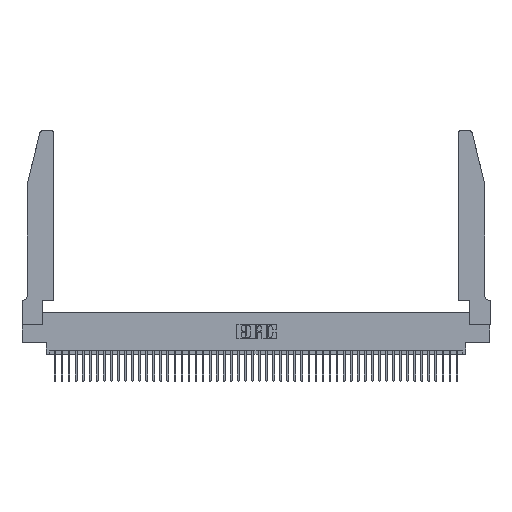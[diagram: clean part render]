
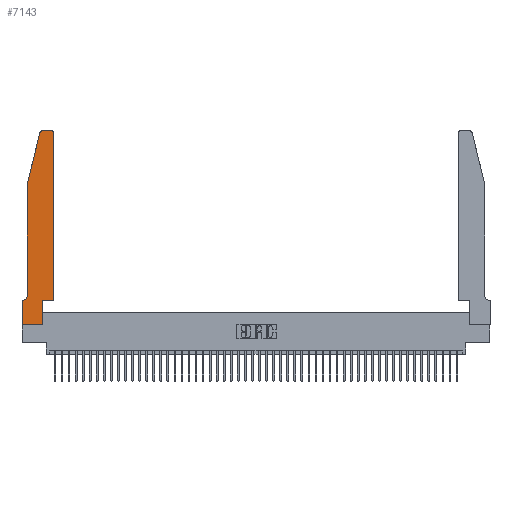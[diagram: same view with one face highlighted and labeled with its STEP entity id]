
A CAD part, top view. The second image highlights one B-rep face of the part: STEP entity #7143.
In plain terms, the highlighted planar face has unit normal (0, 0, 1).
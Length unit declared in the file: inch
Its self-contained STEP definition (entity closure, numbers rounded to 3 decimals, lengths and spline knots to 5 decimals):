
#429 = CARTESIAN_POINT ( 'NONE',  ( 0.4205, 2.75, 0.37 ) ) ;
#1253 = VERTEX_POINT ( 'NONE', #30717 ) ;
#1273 = CIRCLE ( 'NONE', #12332, 0.07 ) ;
#1673 = CARTESIAN_POINT ( 'NONE',  ( 0.0055, 0.42, 0.37 ) ) ;
#1912 = EDGE_CURVE ( 'NONE', #16612, #46207, #1273, .T. ) ;
#2440 = VECTOR ( 'NONE', #19115, 39.37008 ) ;
#2939 = DIRECTION ( 'NONE',  ( 0., -1., 0. ) ) ;
#3280 = CARTESIAN_POINT ( 'NONE',  ( 0.284, 2.75, 0.37 ) ) ;
#4116 = CARTESIAN_POINT ( 'NONE',  ( 0.4505, 0.35, 0.37 ) ) ;
#4199 = CARTESIAN_POINT ( 'NONE',  ( 0.25487, 2.72718, 0.37 ) ) ;
#4573 = EDGE_CURVE ( 'NONE', #17643, #6663, #27404, .T. ) ;
#4672 = EDGE_LOOP ( 'NONE', ( #35767, #28566, #30583, #44725, #23647, #26011, #35428, #19925, #42853, #39651, #7156, #32594 ) ) ;
#5201 = AXIS2_PLACEMENT_3D ( 'NONE', #37118, #32874, #29621 ) ;
#5440 = DIRECTION ( 'NONE',  ( 0., 0., -1. ) ) ;
#6197 = AXIS2_PLACEMENT_3D ( 'NONE', #39773, #47233, #17585 ) ;
#6663 = VERTEX_POINT ( 'NONE', #429 ) ;
#6762 = CARTESIAN_POINT ( 'NONE',  ( 0.2865, 0.35, 0.37 ) ) ;
#7143 = ADVANCED_FACE ( 'NONE', ( #12188 ), #13525, .T. ) ;
#7156 = ORIENTED_EDGE ( 'NONE', *, *, #31594, .T. ) ;
#7603 = DIRECTION ( 'NONE',  ( 1., 0., 0. ) ) ;
#8366 = VECTOR ( 'NONE', #16433, 39.37008 ) ;
#9317 = VECTOR ( 'NONE', #34750, 39.37008 ) ;
#11186 = EDGE_CURVE ( 'NONE', #46207, #47413, #20607, .T. ) ;
#12188 = FACE_OUTER_BOUND ( 'NONE', #4672, .T. ) ;
#12332 = AXIS2_PLACEMENT_3D ( 'NONE', #1673, #5440, #38867 ) ;
#12929 = LINE ( 'NONE', #4116, #2440 ) ;
#13467 = VECTOR ( 'NONE', #36139, 39.37008 ) ;
#13525 = PLANE ( 'NONE',  #6197 ) ;
#13780 = CARTESIAN_POINT ( 'NONE',  ( 0.0055, 0.35, 0.37 ) ) ;
#14168 = VECTOR ( 'NONE', #18924, 39.37008 ) ;
#14359 = CARTESIAN_POINT ( 'NONE',  ( 0., 0., 0.37 ) ) ;
#14623 = DIRECTION ( 'NONE',  ( -1., 0., 0. ) ) ;
#14666 = VERTEX_POINT ( 'NONE', #30146 ) ;
#14786 = CARTESIAN_POINT ( 'NONE',  ( 0.0755, 0.35, 0.37 ) ) ;
#14976 = LINE ( 'NONE', #14359, #25525 ) ;
#15584 = CARTESIAN_POINT ( 'NONE',  ( 0.4505, 2.72, 0.37 ) ) ;
#15757 = EDGE_CURVE ( 'NONE', #42245, #24651, #16914, .T. ) ;
#16433 = DIRECTION ( 'NONE',  ( 1., 0., 0. ) ) ;
#16612 = VERTEX_POINT ( 'NONE', #36038 ) ;
#16914 = LINE ( 'NONE', #26318, #9317 ) ;
#17342 = CARTESIAN_POINT ( 'NONE',  ( 0.0755, 2., 0.37 ) ) ;
#17585 = DIRECTION ( 'NONE',  ( 1., 0., 0. ) ) ;
#17643 = VERTEX_POINT ( 'NONE', #15584 ) ;
#17665 = VECTOR ( 'NONE', #14623, 39.37008 ) ;
#17861 = VECTOR ( 'NONE', #31596, 39.37008 ) ;
#18639 = VECTOR ( 'NONE', #28764, 39.37008 ) ;
#18731 = VERTEX_POINT ( 'NONE', #3280 ) ;
#18924 = DIRECTION ( 'NONE',  ( 0., -1., 0. ) ) ;
#19073 = EDGE_CURVE ( 'NONE', #14666, #42245, #43938, .T. ) ;
#19115 = DIRECTION ( 'NONE',  ( 1., 0., 0. ) ) ;
#19174 = LINE ( 'NONE', #35000, #17861 ) ;
#19593 = EDGE_CURVE ( 'NONE', #6663, #18731, #19174, .T. ) ;
#19721 = CARTESIAN_POINT ( 'NONE',  ( 0., 0., 0.37 ) ) ;
#19925 = ORIENTED_EDGE ( 'NONE', *, *, #19073, .T. ) ;
#20607 = LINE ( 'NONE', #14786, #17665 ) ;
#23597 = EDGE_CURVE ( 'NONE', #36610, #16612, #38091, .T. ) ;
#23647 = ORIENTED_EDGE ( 'NONE', *, *, #1912, .T. ) ;
#24651 = VERTEX_POINT ( 'NONE', #6762 ) ;
#25525 = VECTOR ( 'NONE', #2939, 39.37008 ) ;
#26011 = ORIENTED_EDGE ( 'NONE', *, *, #11186, .T. ) ;
#26318 = CARTESIAN_POINT ( 'NONE',  ( 0.2865, 0.35, 0.37 ) ) ;
#27404 = CIRCLE ( 'NONE', #38605, 0.03 ) ;
#28566 = ORIENTED_EDGE ( 'NONE', *, *, #35561, .T. ) ;
#28571 = LINE ( 'NONE', #17342, #18639 ) ;
#28764 = DIRECTION ( 'NONE',  ( -0.239, -0.971, 0. ) ) ;
#29621 = DIRECTION ( 'NONE',  ( 1., 0., 0. ) ) ;
#29978 = CARTESIAN_POINT ( 'NONE',  ( 0.4205, 2.72, 0.37 ) ) ;
#30146 = CARTESIAN_POINT ( 'NONE',  ( 0., 0., 0.37 ) ) ;
#30583 = ORIENTED_EDGE ( 'NONE', *, *, #41108, .T. ) ;
#30687 = CARTESIAN_POINT ( 'NONE',  ( 0.0755, 2., 0.37 ) ) ;
#30717 = CARTESIAN_POINT ( 'NONE',  ( 0.4505, 0.35, 0.37 ) ) ;
#31594 = EDGE_CURVE ( 'NONE', #1253, #17643, #40272, .T. ) ;
#31596 = DIRECTION ( 'NONE',  ( -1., 0., 0. ) ) ;
#32393 = CARTESIAN_POINT ( 'NONE',  ( 0.4505, 0.35, 0.37 ) ) ;
#32594 = ORIENTED_EDGE ( 'NONE', *, *, #4573, .T. ) ;
#32874 = DIRECTION ( 'NONE',  ( 0., 0., 1. ) ) ;
#34750 = DIRECTION ( 'NONE',  ( 0., 1., 0. ) ) ;
#34786 = CIRCLE ( 'NONE', #5201, 0.03 ) ;
#35000 = CARTESIAN_POINT ( 'NONE',  ( 0.2605, 2.75, 0.37 ) ) ;
#35352 = CARTESIAN_POINT ( 'NONE',  ( 0.2865, 0., 0.37 ) ) ;
#35428 = ORIENTED_EDGE ( 'NONE', *, *, #43652, .T. ) ;
#35561 = EDGE_CURVE ( 'NONE', #18731, #37104, #34786, .T. ) ;
#35767 = ORIENTED_EDGE ( 'NONE', *, *, #19593, .T. ) ;
#36038 = CARTESIAN_POINT ( 'NONE',  ( 0.0755, 0.42, 0.37 ) ) ;
#36139 = DIRECTION ( 'NONE',  ( 0., 1., 0. ) ) ;
#36258 = CARTESIAN_POINT ( 'NONE',  ( 0., 0.35, 0.37 ) ) ;
#36610 = VERTEX_POINT ( 'NONE', #46429 ) ;
#37104 = VERTEX_POINT ( 'NONE', #4199 ) ;
#37118 = CARTESIAN_POINT ( 'NONE',  ( 0.284, 2.72, 0.37 ) ) ;
#37945 = DIRECTION ( 'NONE',  ( 0., 0., 1. ) ) ;
#38091 = LINE ( 'NONE', #30687, #14168 ) ;
#38605 = AXIS2_PLACEMENT_3D ( 'NONE', #29978, #37945, #7603 ) ;
#38867 = DIRECTION ( 'NONE',  ( -1., 0., 0. ) ) ;
#39651 = ORIENTED_EDGE ( 'NONE', *, *, #47711, .T. ) ;
#39773 = CARTESIAN_POINT ( 'NONE',  ( 0., 0.35, 0.37 ) ) ;
#40272 = LINE ( 'NONE', #32393, #13467 ) ;
#41108 = EDGE_CURVE ( 'NONE', #37104, #36610, #28571, .T. ) ;
#42245 = VERTEX_POINT ( 'NONE', #35352 ) ;
#42853 = ORIENTED_EDGE ( 'NONE', *, *, #15757, .T. ) ;
#43652 = EDGE_CURVE ( 'NONE', #47413, #14666, #14976, .T. ) ;
#43938 = LINE ( 'NONE', #19721, #8366 ) ;
#44725 = ORIENTED_EDGE ( 'NONE', *, *, #23597, .T. ) ;
#46207 = VERTEX_POINT ( 'NONE', #13780 ) ;
#46429 = CARTESIAN_POINT ( 'NONE',  ( 0.0755, 2., 0.37 ) ) ;
#47233 = DIRECTION ( 'NONE',  ( 0., 0., 1. ) ) ;
#47413 = VERTEX_POINT ( 'NONE', #36258 ) ;
#47711 = EDGE_CURVE ( 'NONE', #24651, #1253, #12929, .T. ) ;
